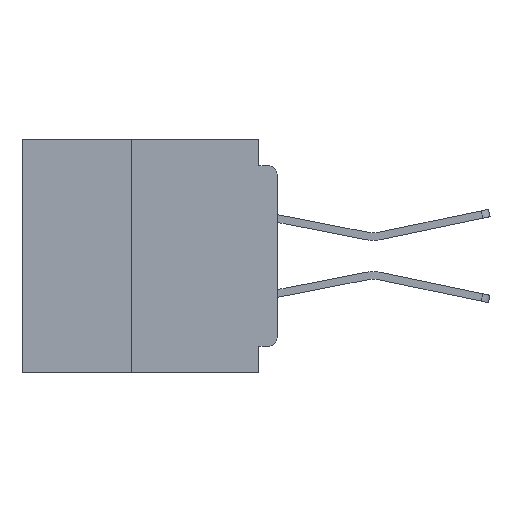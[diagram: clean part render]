
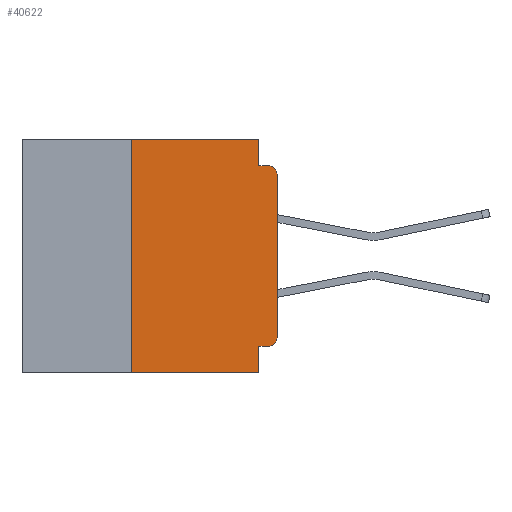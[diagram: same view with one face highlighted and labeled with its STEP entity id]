
A CAD part, left-side view. The second image highlights one B-rep face of the part: STEP entity #40622.
In plain terms, the highlighted planar face has unit normal (-1, 0, 0).
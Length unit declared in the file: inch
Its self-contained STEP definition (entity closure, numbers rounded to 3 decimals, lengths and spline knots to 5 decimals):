
#188 = CARTESIAN_POINT ( 'NONE',  ( 0., 0., -0.34 ) ) ;
#2617 = CARTESIAN_POINT ( 'NONE',  ( 0., 0., -0.06 ) ) ;
#2864 = DIRECTION ( 'NONE',  ( 0., 0., -1. ) ) ;
#3058 = DIRECTION ( 'NONE',  ( 0., 0., -1. ) ) ;
#4087 = LINE ( 'NONE', #49173, #13245 ) ;
#4367 = LINE ( 'NONE', #24607, #35251 ) ;
#5266 = CARTESIAN_POINT ( 'NONE',  ( 0., 0.437, 0. ) ) ;
#5905 = PLANE ( 'NONE',  #16062 ) ;
#6297 = DIRECTION ( 'NONE',  ( 0., 0., 1. ) ) ;
#6786 = CARTESIAN_POINT ( 'NONE',  ( 0., 0., -0.045 ) ) ;
#7376 = EDGE_CURVE ( 'NONE', #43823, #39767, #34575, .T. ) ;
#7573 = LINE ( 'NONE', #29467, #17920 ) ;
#7628 = CARTESIAN_POINT ( 'NONE',  ( 0., 0.437, 0. ) ) ;
#8226 = EDGE_CURVE ( 'NONE', #19014, #26482, #13164, .T. ) ;
#9054 = VERTEX_POINT ( 'NONE', #19520 ) ;
#9199 = DIRECTION ( 'NONE',  ( 0., 0., -1. ) ) ;
#10001 = VECTOR ( 'NONE', #2864, 39.37008 ) ;
#11433 = ORIENTED_EDGE ( 'NONE', *, *, #8226, .F. ) ;
#11917 = VECTOR ( 'NONE', #29936, 39.37008 ) ;
#12147 = VERTEX_POINT ( 'NONE', #38782 ) ;
#13053 = VERTEX_POINT ( 'NONE', #48372 ) ;
#13065 = DIRECTION ( 'NONE',  ( -1., 0., 0. ) ) ;
#13164 = LINE ( 'NONE', #6786, #11917 ) ;
#13245 = VECTOR ( 'NONE', #3058, 39.37008 ) ;
#13345 = CARTESIAN_POINT ( 'NONE',  ( 0., 0.015, -0.34 ) ) ;
#14192 = ORIENTED_EDGE ( 'NONE', *, *, #24034, .T. ) ;
#14992 = EDGE_LOOP ( 'NONE', ( #38551, #14192, #11433, #24249, #42139, #37805, #32946, #45392, #33819, #15762 ) ) ;
#15690 = CARTESIAN_POINT ( 'NONE',  ( 0., 0.25, -0.4 ) ) ;
#15762 = ORIENTED_EDGE ( 'NONE', *, *, #7376, .T. ) ;
#15938 = VECTOR ( 'NONE', #34909, 39.37008 ) ;
#16062 = AXIS2_PLACEMENT_3D ( 'NONE', #5266, #32352, #9199 ) ;
#16330 = EDGE_CURVE ( 'NONE', #13053, #9054, #4367, .T. ) ;
#17261 = DIRECTION ( 'NONE',  ( 0., 0., -1. ) ) ;
#17920 = VECTOR ( 'NONE', #6297, 39.37008 ) ;
#18031 = CARTESIAN_POINT ( 'NONE',  ( 0., 0.25, 0. ) ) ;
#19014 = VERTEX_POINT ( 'NONE', #37602 ) ;
#19345 = DIRECTION ( 'NONE',  ( 0., -1., 0. ) ) ;
#19520 = CARTESIAN_POINT ( 'NONE',  ( 0., 0.031, -0.4 ) ) ;
#19661 = EDGE_CURVE ( 'NONE', #22904, #9054, #4087, .T. ) ;
#22904 = VERTEX_POINT ( 'NONE', #40636 ) ;
#24034 = EDGE_CURVE ( 'NONE', #32846, #26482, #26477, .T. ) ;
#24249 = ORIENTED_EDGE ( 'NONE', *, *, #25438, .F. ) ;
#24502 = VECTOR ( 'NONE', #19345, 39.37008 ) ;
#24607 = CARTESIAN_POINT ( 'NONE',  ( 0., 0.437, -0.4 ) ) ;
#25438 = EDGE_CURVE ( 'NONE', #12147, #19014, #31768, .T. ) ;
#25722 = LINE ( 'NONE', #7628, #24502 ) ;
#26477 = CIRCLE ( 'NONE', #45167, 0.015 ) ;
#26482 = VERTEX_POINT ( 'NONE', #32399 ) ;
#27264 = FACE_OUTER_BOUND ( 'NONE', #14992, .T. ) ;
#28801 = VECTOR ( 'NONE', #47315, 39.37008 ) ;
#29444 = AXIS2_PLACEMENT_3D ( 'NONE', #13345, #40275, #17261 ) ;
#29467 = CARTESIAN_POINT ( 'NONE',  ( 0., 0., 0. ) ) ;
#29936 = DIRECTION ( 'NONE',  ( 0., -1., 0. ) ) ;
#31768 = LINE ( 'NONE', #49001, #10001 ) ;
#32352 = DIRECTION ( 'NONE',  ( 1., 0., 0. ) ) ;
#32394 = DIRECTION ( 'NONE',  ( 0., -1., 0. ) ) ;
#32399 = CARTESIAN_POINT ( 'NONE',  ( 0., 0.015, -0.045 ) ) ;
#32846 = VERTEX_POINT ( 'NONE', #2617 ) ;
#32946 = ORIENTED_EDGE ( 'NONE', *, *, #16330, .T. ) ;
#33819 = ORIENTED_EDGE ( 'NONE', *, *, #43004, .F. ) ;
#34563 = CARTESIAN_POINT ( 'NONE',  ( 0., 0.015, -0.355 ) ) ;
#34575 = CIRCLE ( 'NONE', #29444, 0.015 ) ;
#34909 = DIRECTION ( 'NONE',  ( 0., 0., 1. ) ) ;
#35251 = VECTOR ( 'NONE', #32394, 39.37008 ) ;
#36154 = CARTESIAN_POINT ( 'NONE',  ( 0., 0.015, -0.06 ) ) ;
#37602 = CARTESIAN_POINT ( 'NONE',  ( 0., 0.031, -0.045 ) ) ;
#37609 = LINE ( 'NONE', #15690, #15938 ) ;
#37805 = ORIENTED_EDGE ( 'NONE', *, *, #39759, .F. ) ;
#38266 = EDGE_CURVE ( 'NONE', #39767, #32846, #7573, .T. ) ;
#38551 = ORIENTED_EDGE ( 'NONE', *, *, #38266, .T. ) ;
#38782 = CARTESIAN_POINT ( 'NONE',  ( 0., 0.031, 0. ) ) ;
#39759 = EDGE_CURVE ( 'NONE', #13053, #42580, #37609, .T. ) ;
#39767 = VERTEX_POINT ( 'NONE', #188 ) ;
#40001 = DIRECTION ( 'NONE',  ( 0., 0., -1. ) ) ;
#40275 = DIRECTION ( 'NONE',  ( -1., 0., 0. ) ) ;
#40622 = ADVANCED_FACE ( 'NONE', ( #27264 ), #5905, .F. ) ;
#40636 = CARTESIAN_POINT ( 'NONE',  ( 0., 0.031, -0.355 ) ) ;
#42139 = ORIENTED_EDGE ( 'NONE', *, *, #44408, .F. ) ;
#42580 = VERTEX_POINT ( 'NONE', #18031 ) ;
#43004 = EDGE_CURVE ( 'NONE', #43823, #22904, #49153, .T. ) ;
#43662 = CARTESIAN_POINT ( 'NONE',  ( 0., 0., -0.355 ) ) ;
#43823 = VERTEX_POINT ( 'NONE', #34563 ) ;
#44408 = EDGE_CURVE ( 'NONE', #42580, #12147, #25722, .T. ) ;
#45167 = AXIS2_PLACEMENT_3D ( 'NONE', #36154, #13065, #40001 ) ;
#45392 = ORIENTED_EDGE ( 'NONE', *, *, #19661, .F. ) ;
#47315 = DIRECTION ( 'NONE',  ( 0., 1., 0. ) ) ;
#48372 = CARTESIAN_POINT ( 'NONE',  ( 0., 0.25, -0.4 ) ) ;
#49001 = CARTESIAN_POINT ( 'NONE',  ( 0., 0.031, 0. ) ) ;
#49153 = LINE ( 'NONE', #43662, #28801 ) ;
#49173 = CARTESIAN_POINT ( 'NONE',  ( 0., 0.031, -0.4 ) ) ;
